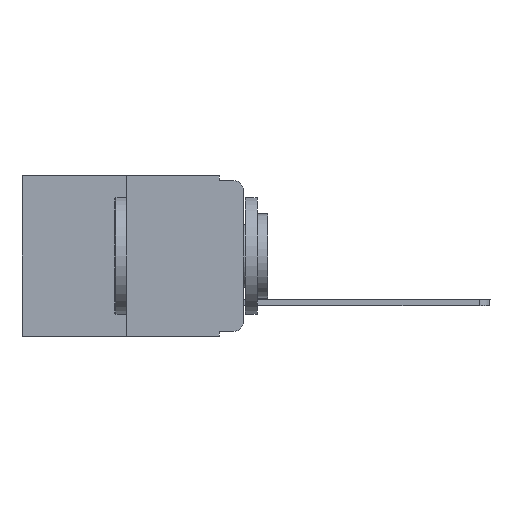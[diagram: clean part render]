
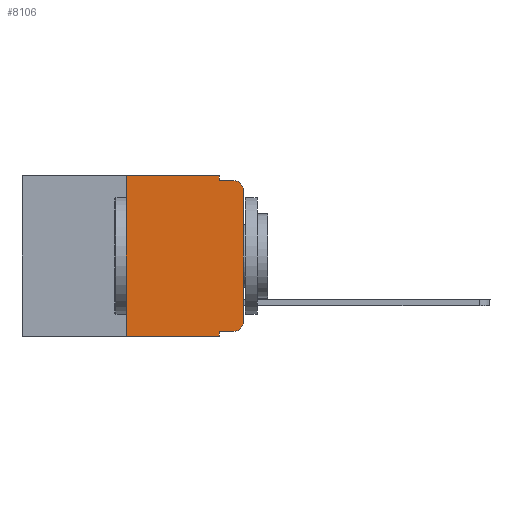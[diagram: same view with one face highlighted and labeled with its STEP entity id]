
A CAD part, left-side view. The second image highlights one B-rep face of the part: STEP entity #8106.
In plain terms, the highlighted planar face has unit normal (-1, 0, 0).
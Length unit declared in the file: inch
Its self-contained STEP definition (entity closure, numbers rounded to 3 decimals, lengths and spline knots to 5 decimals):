
#280 = DIRECTION ( 'NONE',  ( -1., 0., 0. ) ) ;
#360 = CARTESIAN_POINT ( 'NONE',  ( 0., 0., -0.313 ) ) ;
#423 = CIRCLE ( 'NONE', #4210, 0.02 ) ;
#586 = VECTOR ( 'NONE', #12031, 39.37008 ) ;
#706 = CARTESIAN_POINT ( 'NONE',  ( 0., 0., 0. ) ) ;
#877 = VERTEX_POINT ( 'NONE', #7458 ) ;
#1059 = ORIENTED_EDGE ( 'NONE', *, *, #4559, .F. ) ;
#1166 = VERTEX_POINT ( 'NONE', #12430 ) ;
#1628 = VECTOR ( 'NONE', #12853, 39.37008 ) ;
#1736 = CARTESIAN_POINT ( 'NONE',  ( 0., 0., -0.03 ) ) ;
#2133 = CARTESIAN_POINT ( 'NONE',  ( 0., 0.051, 0. ) ) ;
#2249 = VERTEX_POINT ( 'NONE', #360 ) ;
#2556 = VECTOR ( 'NONE', #11249, 39.37008 ) ;
#2578 = VECTOR ( 'NONE', #12340, 39.37008 ) ;
#2750 = EDGE_CURVE ( 'NONE', #1166, #10241, #5213, .T. ) ;
#2775 = LINE ( 'NONE', #2133, #11585 ) ;
#3038 = ORIENTED_EDGE ( 'NONE', *, *, #2750, .F. ) ;
#3088 = ORIENTED_EDGE ( 'NONE', *, *, #3138, .T. ) ;
#3127 = DIRECTION ( 'NONE',  ( 0., 0., -1. ) ) ;
#3138 = EDGE_CURVE ( 'NONE', #6299, #11003, #11077, .T. ) ;
#3706 = VECTOR ( 'NONE', #13362, 39.37008 ) ;
#3724 = CARTESIAN_POINT ( 'NONE',  ( 0., 0.25, -0.343 ) ) ;
#3858 = CARTESIAN_POINT ( 'NONE',  ( 0., 0.051, -0.01 ) ) ;
#4160 = CARTESIAN_POINT ( 'NONE',  ( 0., 0.02, -0.03 ) ) ;
#4210 = AXIS2_PLACEMENT_3D ( 'NONE', #6862, #280, #3127 ) ;
#4217 = PLANE ( 'NONE',  #6520 ) ;
#4320 = DIRECTION ( 'NONE',  ( 1., 0., 0. ) ) ;
#4559 = EDGE_CURVE ( 'NONE', #6299, #10727, #2775, .T. ) ;
#4598 = CARTESIAN_POINT ( 'NONE',  ( 0., 0.473, 0. ) ) ;
#4622 = ORIENTED_EDGE ( 'NONE', *, *, #6296, .T. ) ;
#4816 = DIRECTION ( 'NONE',  ( 0., -1., 0. ) ) ;
#5213 = LINE ( 'NONE', #5402, #586 ) ;
#5302 = EDGE_CURVE ( 'NONE', #6554, #877, #11025, .T. ) ;
#5322 = EDGE_CURVE ( 'NONE', #14154, #1166, #6870, .T. ) ;
#5375 = DIRECTION ( 'NONE',  ( 0., 0., -1. ) ) ;
#5402 = CARTESIAN_POINT ( 'NONE',  ( 0., 0.051, 0. ) ) ;
#5444 = VERTEX_POINT ( 'NONE', #3724 ) ;
#5457 = LINE ( 'NONE', #12156, #2556 ) ;
#5768 = AXIS2_PLACEMENT_3D ( 'NONE', #4160, #6483, #5375 ) ;
#6050 = VECTOR ( 'NONE', #4816, 39.37008 ) ;
#6296 = EDGE_CURVE ( 'NONE', #5444, #10727, #5457, .T. ) ;
#6299 = VERTEX_POINT ( 'NONE', #7934 ) ;
#6483 = DIRECTION ( 'NONE',  ( -1., 0., 0. ) ) ;
#6520 = AXIS2_PLACEMENT_3D ( 'NONE', #8681, #4320, #13083 ) ;
#6554 = VERTEX_POINT ( 'NONE', #1736 ) ;
#6645 = EDGE_LOOP ( 'NONE', ( #12906, #10698, #14210, #3038, #10344, #14158, #4622, #1059, #3088, #12723 ) ) ;
#6862 = CARTESIAN_POINT ( 'NONE',  ( 0., 0.02, -0.313 ) ) ;
#6870 = LINE ( 'NONE', #4598, #2578 ) ;
#7049 = CARTESIAN_POINT ( 'NONE',  ( 0., 0.02, -0.333 ) ) ;
#7378 = CARTESIAN_POINT ( 'NONE',  ( 0., 0.25, 0. ) ) ;
#7458 = CARTESIAN_POINT ( 'NONE',  ( 0., 0.02, -0.01 ) ) ;
#7869 = EDGE_CURVE ( 'NONE', #11003, #2249, #423, .T. ) ;
#7934 = CARTESIAN_POINT ( 'NONE',  ( 0., 0.051, -0.333 ) ) ;
#8066 = EDGE_CURVE ( 'NONE', #10241, #877, #11472, .T. ) ;
#8106 = ADVANCED_FACE ( 'NONE', ( #10761 ), #4217, .F. ) ;
#8681 = CARTESIAN_POINT ( 'NONE',  ( 0., 0.473, 0. ) ) ;
#9735 = LINE ( 'NONE', #706, #1628 ) ;
#10084 = CARTESIAN_POINT ( 'NONE',  ( 0., 0.25, 0. ) ) ;
#10241 = VERTEX_POINT ( 'NONE', #3858 ) ;
#10344 = ORIENTED_EDGE ( 'NONE', *, *, #5322, .F. ) ;
#10623 = LINE ( 'NONE', #10084, #3706 ) ;
#10662 = CARTESIAN_POINT ( 'NONE',  ( 0., 0.051, -0.343 ) ) ;
#10698 = ORIENTED_EDGE ( 'NONE', *, *, #5302, .T. ) ;
#10727 = VERTEX_POINT ( 'NONE', #10662 ) ;
#10761 = FACE_OUTER_BOUND ( 'NONE', #6645, .T. ) ;
#11003 = VERTEX_POINT ( 'NONE', #7049 ) ;
#11025 = CIRCLE ( 'NONE', #5768, 0.02 ) ;
#11077 = LINE ( 'NONE', #11449, #6050 ) ;
#11093 = DIRECTION ( 'NONE',  ( 0., 0., -1. ) ) ;
#11105 = VECTOR ( 'NONE', #11786, 39.37008 ) ;
#11249 = DIRECTION ( 'NONE',  ( 0., -1., 0. ) ) ;
#11358 = EDGE_CURVE ( 'NONE', #5444, #14154, #10623, .T. ) ;
#11449 = CARTESIAN_POINT ( 'NONE',  ( 0., 0.051, -0.333 ) ) ;
#11472 = LINE ( 'NONE', #14143, #11105 ) ;
#11585 = VECTOR ( 'NONE', #11093, 39.37008 ) ;
#11786 = DIRECTION ( 'NONE',  ( 0., -1., 0. ) ) ;
#12031 = DIRECTION ( 'NONE',  ( 0., 0., -1. ) ) ;
#12156 = CARTESIAN_POINT ( 'NONE',  ( 0., 0.473, -0.343 ) ) ;
#12337 = EDGE_CURVE ( 'NONE', #2249, #6554, #9735, .T. ) ;
#12340 = DIRECTION ( 'NONE',  ( 0., -1., 0. ) ) ;
#12430 = CARTESIAN_POINT ( 'NONE',  ( 0., 0.051, 0. ) ) ;
#12723 = ORIENTED_EDGE ( 'NONE', *, *, #7869, .T. ) ;
#12853 = DIRECTION ( 'NONE',  ( 0., 0., 1. ) ) ;
#12906 = ORIENTED_EDGE ( 'NONE', *, *, #12337, .T. ) ;
#13083 = DIRECTION ( 'NONE',  ( 0., 0., -1. ) ) ;
#13362 = DIRECTION ( 'NONE',  ( 0., 0., 1. ) ) ;
#14143 = CARTESIAN_POINT ( 'NONE',  ( 0., 0.051, -0.01 ) ) ;
#14154 = VERTEX_POINT ( 'NONE', #7378 ) ;
#14158 = ORIENTED_EDGE ( 'NONE', *, *, #11358, .F. ) ;
#14210 = ORIENTED_EDGE ( 'NONE', *, *, #8066, .F. ) ;
